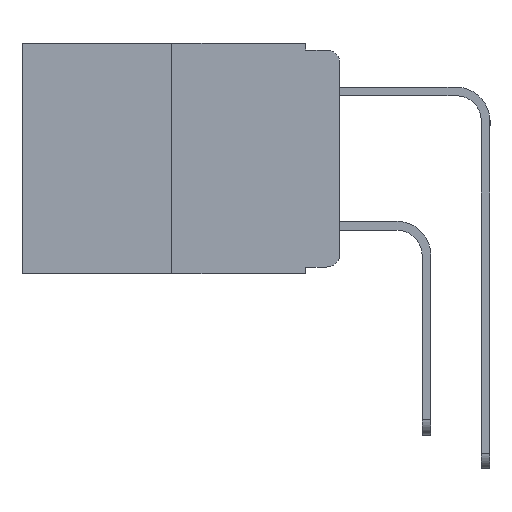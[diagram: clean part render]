
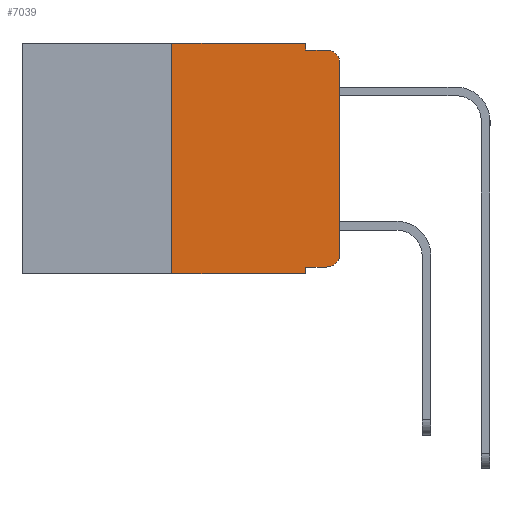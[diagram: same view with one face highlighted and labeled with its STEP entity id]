
A CAD part, left-side view. The second image highlights one B-rep face of the part: STEP entity #7039.
In plain terms, the highlighted planar face has unit normal (-1, 0, 0).
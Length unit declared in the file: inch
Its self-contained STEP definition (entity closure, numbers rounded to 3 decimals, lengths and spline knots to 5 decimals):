
#66 = VERTEX_POINT ( 'NONE', #3234 ) ;
#102 = CARTESIAN_POINT ( 'NONE',  ( 0., 0.051, -0.01 ) ) ;
#118 = VECTOR ( 'NONE', #13066, 39.37008 ) ;
#285 = DIRECTION ( 'NONE',  ( 0., 0., -1. ) ) ;
#339 = ORIENTED_EDGE ( 'NONE', *, *, #7159, .T. ) ;
#819 = EDGE_CURVE ( 'NONE', #11463, #10567, #11731, .T. ) ;
#860 = CARTESIAN_POINT ( 'NONE',  ( 0., 0.051, -0.01 ) ) ;
#1078 = LINE ( 'NONE', #11944, #118 ) ;
#1202 = VECTOR ( 'NONE', #14429, 39.37008 ) ;
#1503 = CIRCLE ( 'NONE', #9181, 0.02 ) ;
#1586 = DIRECTION ( 'NONE',  ( 0., -1., 0. ) ) ;
#2071 = CARTESIAN_POINT ( 'NONE',  ( 0., 0.02, -0.01 ) ) ;
#2129 = VERTEX_POINT ( 'NONE', #12649 ) ;
#2566 = ORIENTED_EDGE ( 'NONE', *, *, #7111, .F. ) ;
#2798 = EDGE_CURVE ( 'NONE', #2129, #66, #4464, .T. ) ;
#3055 = ORIENTED_EDGE ( 'NONE', *, *, #7110, .F. ) ;
#3187 = VECTOR ( 'NONE', #1586, 39.37008 ) ;
#3234 = CARTESIAN_POINT ( 'NONE',  ( 0., 0.051, -0.343 ) ) ;
#3895 = DIRECTION ( 'NONE',  ( 0., -1., 0. ) ) ;
#4179 = VERTEX_POINT ( 'NONE', #9816 ) ;
#4464 = LINE ( 'NONE', #6561, #1202 ) ;
#4872 = ORIENTED_EDGE ( 'NONE', *, *, #7093, .T. ) ;
#5029 = DIRECTION ( 'NONE',  ( 1., 0., 0. ) ) ;
#5143 = VERTEX_POINT ( 'NONE', #13990 ) ;
#5514 = VECTOR ( 'NONE', #3895, 39.37008 ) ;
#5630 = CARTESIAN_POINT ( 'NONE',  ( 0., 0.25, 0. ) ) ;
#5944 = DIRECTION ( 'NONE',  ( 0., -1., 0. ) ) ;
#6179 = ORIENTED_EDGE ( 'NONE', *, *, #2798, .T. ) ;
#6316 = CARTESIAN_POINT ( 'NONE',  ( 0., 0.02, -0.03 ) ) ;
#6347 = VECTOR ( 'NONE', #7514, 39.37008 ) ;
#6359 = CARTESIAN_POINT ( 'NONE',  ( 0., 0.25, 0. ) ) ;
#6561 = CARTESIAN_POINT ( 'NONE',  ( 0., 0.473, -0.343 ) ) ;
#6786 = ORIENTED_EDGE ( 'NONE', *, *, #7130, .F. ) ;
#7039 = ADVANCED_FACE ( 'NONE', ( #8907 ), #7327, .F. ) ;
#7090 = EDGE_CURVE ( 'NONE', #7913, #5143, #7838, .T. ) ;
#7093 = EDGE_CURVE ( 'NONE', #5143, #10312, #1503, .T. ) ;
#7110 = EDGE_CURVE ( 'NONE', #8033, #10312, #13398, .T. ) ;
#7111 = EDGE_CURVE ( 'NONE', #10567, #8033, #1078, .T. ) ;
#7114 = EDGE_CURVE ( 'NONE', #2129, #11463, #9407, .T. ) ;
#7130 = EDGE_CURVE ( 'NONE', #10458, #66, #9048, .T. ) ;
#7138 = EDGE_CURVE ( 'NONE', #10458, #4179, #12318, .T. ) ;
#7159 = EDGE_CURVE ( 'NONE', #4179, #7913, #8688, .T. ) ;
#7327 = PLANE ( 'NONE',  #8424 ) ;
#7411 = ORIENTED_EDGE ( 'NONE', *, *, #7090, .T. ) ;
#7467 = DIRECTION ( 'NONE',  ( 0., 0., -1. ) ) ;
#7514 = DIRECTION ( 'NONE',  ( 0., 0., 1. ) ) ;
#7572 = CARTESIAN_POINT ( 'NONE',  ( 0., 0.051, -0.333 ) ) ;
#7617 = DIRECTION ( 'NONE',  ( -1., 0., 0. ) ) ;
#7642 = AXIS2_PLACEMENT_3D ( 'NONE', #14263, #7617, #285 ) ;
#7660 = EDGE_LOOP ( 'NONE', ( #7411, #4872, #3055, #2566, #9988, #10408, #6179, #6786, #7710, #339 ) ) ;
#7710 = ORIENTED_EDGE ( 'NONE', *, *, #7138, .T. ) ;
#7838 = LINE ( 'NONE', #14081, #10493 ) ;
#7913 = VERTEX_POINT ( 'NONE', #11274 ) ;
#8033 = VERTEX_POINT ( 'NONE', #860 ) ;
#8246 = CARTESIAN_POINT ( 'NONE',  ( 0., 0.051, -0.333 ) ) ;
#8424 = AXIS2_PLACEMENT_3D ( 'NONE', #10748, #5029, #12922 ) ;
#8688 = CIRCLE ( 'NONE', #7642, 0.02 ) ;
#8907 = FACE_OUTER_BOUND ( 'NONE', #7660, .T. ) ;
#9048 = LINE ( 'NONE', #10928, #11952 ) ;
#9181 = AXIS2_PLACEMENT_3D ( 'NONE', #6316, #14133, #7467 ) ;
#9407 = LINE ( 'NONE', #6359, #6347 ) ;
#9816 = CARTESIAN_POINT ( 'NONE',  ( 0., 0.02, -0.333 ) ) ;
#9977 = CARTESIAN_POINT ( 'NONE',  ( 0., 0.473, 0. ) ) ;
#9988 = ORIENTED_EDGE ( 'NONE', *, *, #819, .F. ) ;
#10312 = VERTEX_POINT ( 'NONE', #2071 ) ;
#10408 = ORIENTED_EDGE ( 'NONE', *, *, #7114, .F. ) ;
#10458 = VERTEX_POINT ( 'NONE', #8246 ) ;
#10493 = VECTOR ( 'NONE', #10831, 39.37008 ) ;
#10567 = VERTEX_POINT ( 'NONE', #13939 ) ;
#10748 = CARTESIAN_POINT ( 'NONE',  ( 0., 0.473, 0. ) ) ;
#10831 = DIRECTION ( 'NONE',  ( 0., 0., 1. ) ) ;
#10928 = CARTESIAN_POINT ( 'NONE',  ( 0., 0.051, 0. ) ) ;
#11274 = CARTESIAN_POINT ( 'NONE',  ( 0., 0., -0.313 ) ) ;
#11397 = VECTOR ( 'NONE', #5944, 39.37008 ) ;
#11463 = VERTEX_POINT ( 'NONE', #5630 ) ;
#11731 = LINE ( 'NONE', #9977, #11397 ) ;
#11944 = CARTESIAN_POINT ( 'NONE',  ( 0., 0.051, 0. ) ) ;
#11952 = VECTOR ( 'NONE', #11983, 39.37008 ) ;
#11983 = DIRECTION ( 'NONE',  ( 0., 0., -1. ) ) ;
#12318 = LINE ( 'NONE', #7572, #3187 ) ;
#12649 = CARTESIAN_POINT ( 'NONE',  ( 0., 0.25, -0.343 ) ) ;
#12922 = DIRECTION ( 'NONE',  ( 0., 0., -1. ) ) ;
#13066 = DIRECTION ( 'NONE',  ( 0., 0., -1. ) ) ;
#13398 = LINE ( 'NONE', #102, #5514 ) ;
#13939 = CARTESIAN_POINT ( 'NONE',  ( 0., 0.051, 0. ) ) ;
#13990 = CARTESIAN_POINT ( 'NONE',  ( 0., 0., -0.03 ) ) ;
#14081 = CARTESIAN_POINT ( 'NONE',  ( 0., 0., 0. ) ) ;
#14133 = DIRECTION ( 'NONE',  ( -1., 0., 0. ) ) ;
#14263 = CARTESIAN_POINT ( 'NONE',  ( 0., 0.02, -0.313 ) ) ;
#14429 = DIRECTION ( 'NONE',  ( 0., -1., 0. ) ) ;
